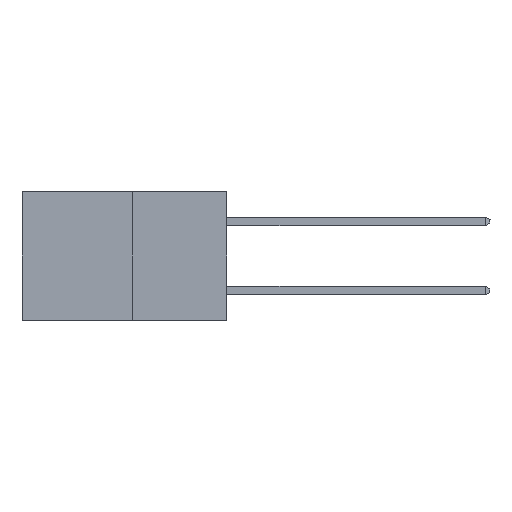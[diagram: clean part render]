
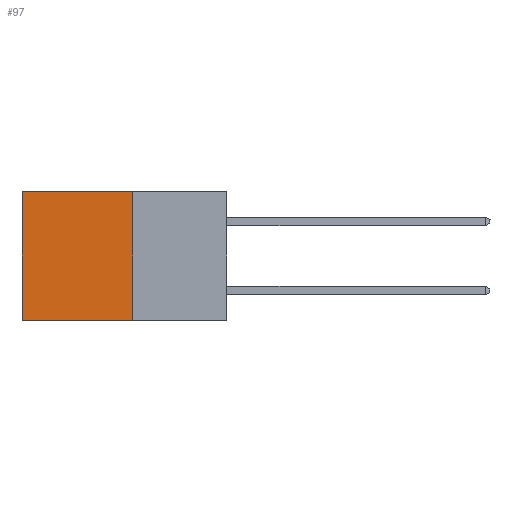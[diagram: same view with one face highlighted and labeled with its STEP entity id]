
A CAD part, left-side view. The second image highlights one B-rep face of the part: STEP entity #97.
In plain terms, the highlighted planar face has unit normal (-1, 0, 0).
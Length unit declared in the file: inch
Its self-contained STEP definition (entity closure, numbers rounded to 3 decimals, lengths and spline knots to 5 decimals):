
#4 = ORIENTED_EDGE ( 'NONE', *, *, #1976, .T. ) ;
#19 = ORIENTED_EDGE ( 'NONE', *, *, #4168, .F. ) ;
#53 = ORIENTED_EDGE ( 'NONE', *, *, #8665, .F. ) ;
#66 = ORIENTED_EDGE ( 'NONE', *, *, #7286, .T. ) ;
#97 = ADVANCED_FACE ( 'NONE', ( #4573 ), #1453, .F. ) ;
#300 = LINE ( 'NONE', #3361, #6783 ) ;
#375 = CARTESIAN_POINT ( 'NONE',  ( 0.277, 0.59, -0.37 ) ) ;
#595 = DIRECTION ( 'NONE',  ( 1., 0., 0. ) ) ;
#654 = VERTEX_POINT ( 'NONE', #6522 ) ;
#1303 = VECTOR ( 'NONE', #9231, 39.37008 ) ;
#1382 = AXIS2_PLACEMENT_3D ( 'NONE', #3130, #595, #9024 ) ;
#1453 = PLANE ( 'NONE',  #1382 ) ;
#1503 = VECTOR ( 'NONE', #9847, 39.37008 ) ;
#1730 = CARTESIAN_POINT ( 'NONE',  ( 0.277, 0.27, 0. ) ) ;
#1976 = EDGE_CURVE ( 'NONE', #8846, #7702, #9868, .T. ) ;
#3130 = CARTESIAN_POINT ( 'NONE',  ( 0.277, 0.27, -0.37 ) ) ;
#3361 = CARTESIAN_POINT ( 'NONE',  ( 0.277, 0.27, -0.37 ) ) ;
#4168 = EDGE_CURVE ( 'NONE', #5786, #7702, #300, .T. ) ;
#4365 = VECTOR ( 'NONE', #8026, 39.37008 ) ;
#4573 = FACE_OUTER_BOUND ( 'NONE', #10381, .T. ) ;
#5744 = DIRECTION ( 'NONE',  ( 0., 1., 0. ) ) ;
#5786 = VERTEX_POINT ( 'NONE', #7450 ) ;
#5971 = LINE ( 'NONE', #1730, #4365 ) ;
#6522 = CARTESIAN_POINT ( 'NONE',  ( 0.277, 0.27, 0. ) ) ;
#6783 = VECTOR ( 'NONE', #5744, 39.37008 ) ;
#6926 = CARTESIAN_POINT ( 'NONE',  ( 0.277, 0.27, -0.37 ) ) ;
#7286 = EDGE_CURVE ( 'NONE', #654, #8846, #5971, .T. ) ;
#7450 = CARTESIAN_POINT ( 'NONE',  ( 0.277, 0.27, -0.37 ) ) ;
#7702 = VERTEX_POINT ( 'NONE', #375 ) ;
#7872 = CARTESIAN_POINT ( 'NONE',  ( 0.277, 0.59, 0. ) ) ;
#8026 = DIRECTION ( 'NONE',  ( 0., 1., 0. ) ) ;
#8064 = CARTESIAN_POINT ( 'NONE',  ( 0.277, 0.59, -0.37 ) ) ;
#8665 = EDGE_CURVE ( 'NONE', #654, #5786, #9697, .T. ) ;
#8846 = VERTEX_POINT ( 'NONE', #7872 ) ;
#9024 = DIRECTION ( 'NONE',  ( 0., 0., -1. ) ) ;
#9231 = DIRECTION ( 'NONE',  ( 0., 0., -1. ) ) ;
#9697 = LINE ( 'NONE', #6926, #1303 ) ;
#9847 = DIRECTION ( 'NONE',  ( 0., 0., -1. ) ) ;
#9868 = LINE ( 'NONE', #8064, #1503 ) ;
#10381 = EDGE_LOOP ( 'NONE', ( #4, #19, #53, #66 ) ) ;
